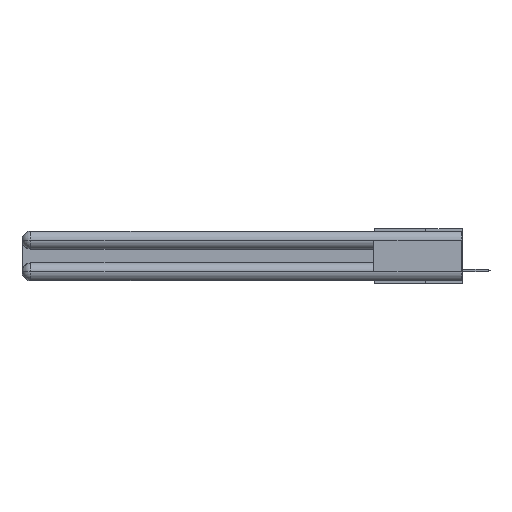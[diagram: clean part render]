
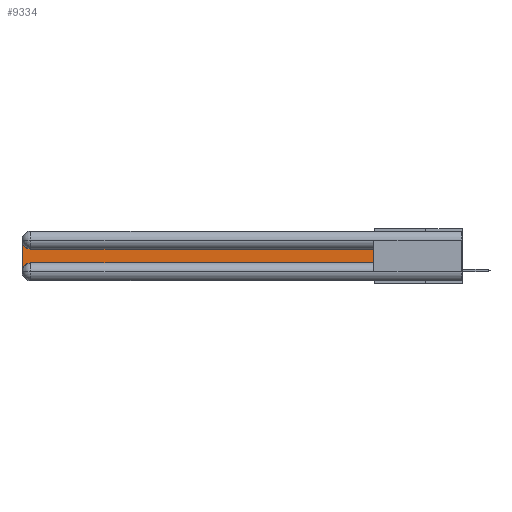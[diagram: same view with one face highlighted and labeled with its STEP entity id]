
A CAD part, left-side view. The second image highlights one B-rep face of the part: STEP entity #9334.
In plain terms, the highlighted planar face has unit normal (-1, 0, 0).
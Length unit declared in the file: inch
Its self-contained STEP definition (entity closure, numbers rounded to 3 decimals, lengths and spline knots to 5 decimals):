
#90 = ORIENTED_EDGE ( 'NONE', *, *, #16454, .T. ) ;
#191 = VECTOR ( 'NONE', #16401, 39.37008 ) ;
#833 = VERTEX_POINT ( 'NONE', #19069 ) ;
#1317 = EDGE_LOOP ( 'NONE', ( #90, #28644, #24201, #22370, #24315, #30157 ) ) ;
#1425 = CARTESIAN_POINT ( 'NONE',  ( 0.075, 2.94, -0.0625 ) ) ;
#1446 = CARTESIAN_POINT ( 'NONE',  ( 0.075, 0.6, -0.1225 ) ) ;
#1544 = DIRECTION ( 'NONE',  ( 1., 0., 0. ) ) ;
#4914 = CARTESIAN_POINT ( 'NONE',  ( 0.075, 0.6, -0.1225 ) ) ;
#5137 = EDGE_CURVE ( 'NONE', #30481, #833, #6933, .T. ) ;
#6933 = CIRCLE ( 'NONE', #20097, 0.06 ) ;
#7192 = LINE ( 'NONE', #21436, #18763 ) ;
#8754 = CIRCLE ( 'NONE', #20408, 0.06 ) ;
#8875 = DIRECTION ( 'NONE',  ( 0., -1., 0. ) ) ;
#9286 = CARTESIAN_POINT ( 'NONE',  ( 0.075, 3., -0.1225 ) ) ;
#9334 = ADVANCED_FACE ( 'NONE', ( #14761 ), #29345, .F. ) ;
#11124 = LINE ( 'NONE', #4914, #21954 ) ;
#11321 = CARTESIAN_POINT ( 'NONE',  ( 0.075, 0.6, -0.2175 ) ) ;
#12257 = DIRECTION ( 'NONE',  ( 1., 0., 0. ) ) ;
#12479 = DIRECTION ( 'NONE',  ( 0., 0., -1. ) ) ;
#14761 = FACE_OUTER_BOUND ( 'NONE', #1317, .T. ) ;
#14967 = DIRECTION ( 'NONE',  ( 0., 1., 0. ) ) ;
#16180 = VERTEX_POINT ( 'NONE', #11321 ) ;
#16401 = DIRECTION ( 'NONE',  ( 0., 0., 1. ) ) ;
#16454 = EDGE_CURVE ( 'NONE', #19835, #30481, #11124, .T. ) ;
#16772 = EDGE_CURVE ( 'NONE', #30549, #16180, #7192, .T. ) ;
#18763 = VECTOR ( 'NONE', #8875, 39.37008 ) ;
#18803 = DIRECTION ( 'NONE',  ( 0., 0., -1. ) ) ;
#19069 = CARTESIAN_POINT ( 'NONE',  ( 0.075, 3., -0.0625 ) ) ;
#19209 = DIRECTION ( 'NONE',  ( 1., 0., 0. ) ) ;
#19835 = VERTEX_POINT ( 'NONE', #1446 ) ;
#20097 = AXIS2_PLACEMENT_3D ( 'NONE', #1425, #1544, #18803 ) ;
#20408 = AXIS2_PLACEMENT_3D ( 'NONE', #31993, #12257, #12479 ) ;
#21373 = CARTESIAN_POINT ( 'NONE',  ( 0.075, 2.94, -0.2175 ) ) ;
#21436 = CARTESIAN_POINT ( 'NONE',  ( 0.075, 0.6, -0.2175 ) ) ;
#21954 = VECTOR ( 'NONE', #14967, 39.37008 ) ;
#22370 = ORIENTED_EDGE ( 'NONE', *, *, #31457, .T. ) ;
#22513 = EDGE_CURVE ( 'NONE', #16180, #19835, #29230, .T. ) ;
#23310 = AXIS2_PLACEMENT_3D ( 'NONE', #9286, #19209, #29240 ) ;
#23481 = CARTESIAN_POINT ( 'NONE',  ( 0.075, 0.6, -0.2175 ) ) ;
#23935 = VECTOR ( 'NONE', #25699, 39.37008 ) ;
#24201 = ORIENTED_EDGE ( 'NONE', *, *, #30975, .T. ) ;
#24315 = ORIENTED_EDGE ( 'NONE', *, *, #16772, .T. ) ;
#24839 = CARTESIAN_POINT ( 'NONE',  ( 0.075, 3., -0.2775 ) ) ;
#25699 = DIRECTION ( 'NONE',  ( 0., 0., -1. ) ) ;
#25912 = CARTESIAN_POINT ( 'NONE',  ( 0.075, 3., -0.2175 ) ) ;
#25950 = CARTESIAN_POINT ( 'NONE',  ( 0.075, 2.94, -0.1225 ) ) ;
#26276 = LINE ( 'NONE', #25912, #23935 ) ;
#28644 = ORIENTED_EDGE ( 'NONE', *, *, #5137, .T. ) ;
#29230 = LINE ( 'NONE', #23481, #191 ) ;
#29240 = DIRECTION ( 'NONE',  ( 0., 0., -1. ) ) ;
#29345 = PLANE ( 'NONE',  #23310 ) ;
#30157 = ORIENTED_EDGE ( 'NONE', *, *, #22513, .T. ) ;
#30481 = VERTEX_POINT ( 'NONE', #25950 ) ;
#30549 = VERTEX_POINT ( 'NONE', #21373 ) ;
#30739 = VERTEX_POINT ( 'NONE', #24839 ) ;
#30975 = EDGE_CURVE ( 'NONE', #833, #30739, #26276, .T. ) ;
#31457 = EDGE_CURVE ( 'NONE', #30739, #30549, #8754, .T. ) ;
#31993 = CARTESIAN_POINT ( 'NONE',  ( 0.075, 2.94, -0.2775 ) ) ;
